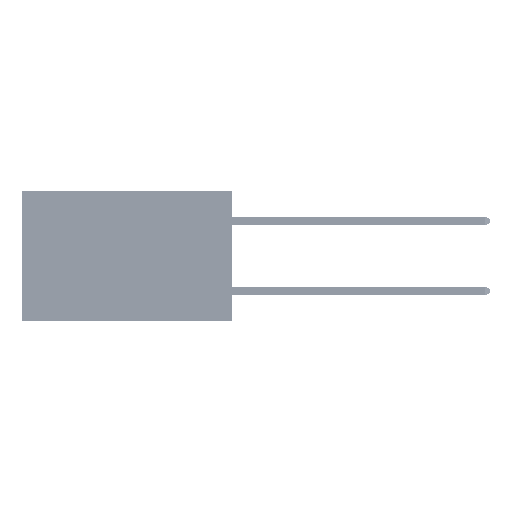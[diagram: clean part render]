
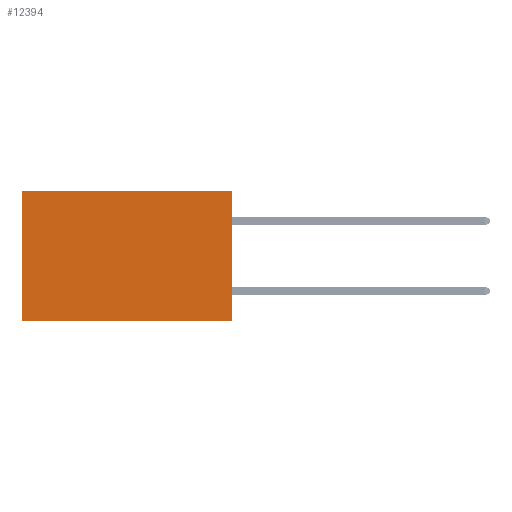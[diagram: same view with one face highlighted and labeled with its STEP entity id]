
A CAD part, left-side view. The second image highlights one B-rep face of the part: STEP entity #12394.
In plain terms, the highlighted planar face has unit normal (-1, 0, 0).
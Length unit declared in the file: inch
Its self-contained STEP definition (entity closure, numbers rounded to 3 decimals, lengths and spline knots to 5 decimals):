
#382 = EDGE_CURVE ( 'NONE', #29423, #12166, #23296, .T. ) ;
#1624 = LINE ( 'NONE', #40832, #2217 ) ;
#2217 = VECTOR ( 'NONE', #36550, 39.37008 ) ;
#2339 = VERTEX_POINT ( 'NONE', #5687 ) ;
#2816 = ORIENTED_EDGE ( 'NONE', *, *, #17991, .T. ) ;
#3219 = ORIENTED_EDGE ( 'NONE', *, *, #35152, .F. ) ;
#3856 = ORIENTED_EDGE ( 'NONE', *, *, #382, .F. ) ;
#5496 = VECTOR ( 'NONE', #30266, 39.37008 ) ;
#5687 = CARTESIAN_POINT ( 'NONE',  ( 0.2875, 0.6, -0.37 ) ) ;
#6485 = CARTESIAN_POINT ( 'NONE',  ( 0.2875, 0., 0. ) ) ;
#7611 = DIRECTION ( 'NONE',  ( 0., 1., 0. ) ) ;
#11275 = CARTESIAN_POINT ( 'NONE',  ( 0.2875, 0., 0. ) ) ;
#12166 = VERTEX_POINT ( 'NONE', #46381 ) ;
#12394 = ADVANCED_FACE ( 'NONE', ( #40034 ), #28733, .F. ) ;
#12884 = VECTOR ( 'NONE', #7611, 39.37008 ) ;
#13165 = DIRECTION ( 'NONE',  ( 0., 0., -1. ) ) ;
#14711 = LINE ( 'NONE', #31763, #12884 ) ;
#15809 = LINE ( 'NONE', #11275, #40874 ) ;
#17991 = EDGE_CURVE ( 'NONE', #25586, #2339, #1624, .T. ) ;
#20249 = EDGE_CURVE ( 'NONE', #29423, #25586, #15809, .T. ) ;
#23296 = LINE ( 'NONE', #29942, #5496 ) ;
#25334 = DIRECTION ( 'NONE',  ( 1., 0., 0. ) ) ;
#25586 = VERTEX_POINT ( 'NONE', #35270 ) ;
#28733 = PLANE ( 'NONE',  #40519 ) ;
#29423 = VERTEX_POINT ( 'NONE', #6485 ) ;
#29942 = CARTESIAN_POINT ( 'NONE',  ( 0.2875, 0., 0. ) ) ;
#30266 = DIRECTION ( 'NONE',  ( 0., 0., -1. ) ) ;
#31763 = CARTESIAN_POINT ( 'NONE',  ( 0.2875, 0., -0.37 ) ) ;
#32398 = ORIENTED_EDGE ( 'NONE', *, *, #20249, .T. ) ;
#35152 = EDGE_CURVE ( 'NONE', #12166, #2339, #14711, .T. ) ;
#35270 = CARTESIAN_POINT ( 'NONE',  ( 0.2875, 0.6, 0. ) ) ;
#36141 = EDGE_LOOP ( 'NONE', ( #2816, #3219, #3856, #32398 ) ) ;
#36550 = DIRECTION ( 'NONE',  ( 0., 0., -1. ) ) ;
#40034 = FACE_OUTER_BOUND ( 'NONE', #36141, .T. ) ;
#40519 = AXIS2_PLACEMENT_3D ( 'NONE', #44793, #25334, #13165 ) ;
#40832 = CARTESIAN_POINT ( 'NONE',  ( 0.2875, 0.6, 0. ) ) ;
#40874 = VECTOR ( 'NONE', #50626, 39.37008 ) ;
#44793 = CARTESIAN_POINT ( 'NONE',  ( 0.2875, 0., 0. ) ) ;
#46381 = CARTESIAN_POINT ( 'NONE',  ( 0.2875, 0., -0.37 ) ) ;
#50626 = DIRECTION ( 'NONE',  ( 0., 1., 0. ) ) ;
